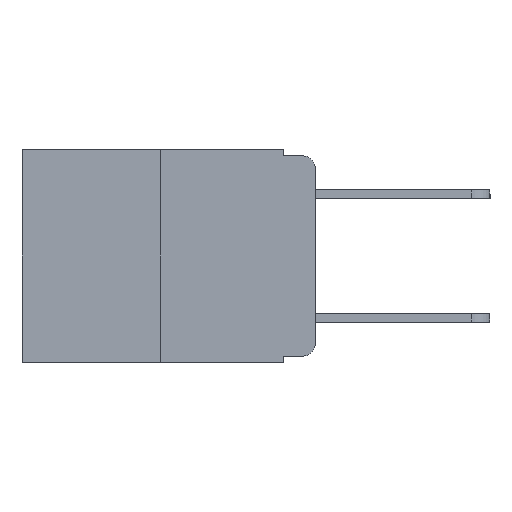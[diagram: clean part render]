
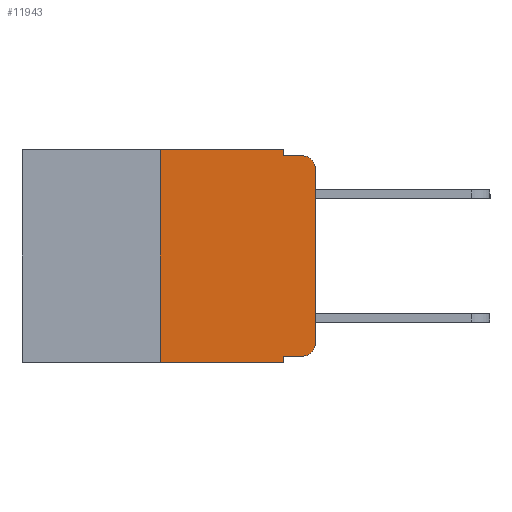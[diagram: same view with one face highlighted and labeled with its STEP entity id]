
A CAD part, left-side view. The second image highlights one B-rep face of the part: STEP entity #11943.
In plain terms, the highlighted planar face has unit normal (-1, 0, 0).
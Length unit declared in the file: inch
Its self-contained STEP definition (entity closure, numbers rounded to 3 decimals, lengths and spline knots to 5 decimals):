
#46 = ORIENTED_EDGE ( 'NONE', *, *, #11764, .F. ) ;
#223 = CARTESIAN_POINT ( 'NONE',  ( 0., 0.02, -0.313 ) ) ;
#431 = CARTESIAN_POINT ( 'NONE',  ( 0., 0.25, 0. ) ) ;
#794 = DIRECTION ( 'NONE',  ( -1., 0., 0. ) ) ;
#873 = ORIENTED_EDGE ( 'NONE', *, *, #11497, .T. ) ;
#1015 = CARTESIAN_POINT ( 'NONE',  ( 0., 0.051, -0.333 ) ) ;
#1298 = DIRECTION ( 'NONE',  ( 0., 0., -1. ) ) ;
#1335 = DIRECTION ( 'NONE',  ( 1., 0., 0. ) ) ;
#1840 = CARTESIAN_POINT ( 'NONE',  ( 0., 0.051, -0.01 ) ) ;
#1846 = ORIENTED_EDGE ( 'NONE', *, *, #12271, .F. ) ;
#1967 = VERTEX_POINT ( 'NONE', #11805 ) ;
#2085 = VERTEX_POINT ( 'NONE', #2426 ) ;
#2142 = VECTOR ( 'NONE', #12217, 39.37008 ) ;
#2426 = CARTESIAN_POINT ( 'NONE',  ( 0., 0.02, -0.333 ) ) ;
#2432 = VERTEX_POINT ( 'NONE', #2694 ) ;
#2457 = CARTESIAN_POINT ( 'NONE',  ( 0., 0.051, -0.333 ) ) ;
#2475 = LINE ( 'NONE', #9108, #10427 ) ;
#2492 = CARTESIAN_POINT ( 'NONE',  ( 0., 0.25, -0.343 ) ) ;
#2615 = EDGE_CURVE ( 'NONE', #10436, #3575, #9193, .T. ) ;
#2694 = CARTESIAN_POINT ( 'NONE',  ( 0., 0.02, -0.01 ) ) ;
#2978 = LINE ( 'NONE', #10700, #7921 ) ;
#3047 = VECTOR ( 'NONE', #7448, 39.37008 ) ;
#3259 = EDGE_CURVE ( 'NONE', #6169, #12086, #2475, .T. ) ;
#3275 = EDGE_CURVE ( 'NONE', #6140, #1967, #9878, .T. ) ;
#3575 = VERTEX_POINT ( 'NONE', #10902 ) ;
#3924 = EDGE_LOOP ( 'NONE', ( #873, #11348, #1846, #7428, #46, #10440, #8321, #6031, #8918, #6675 ) ) ;
#4031 = DIRECTION ( 'NONE',  ( 0., -1., 0. ) ) ;
#4522 = DIRECTION ( 'NONE',  ( 0., 0., -1. ) ) ;
#4551 = EDGE_CURVE ( 'NONE', #6140, #2085, #8284, .T. ) ;
#4574 = CARTESIAN_POINT ( 'NONE',  ( 0., 0.473, -0.343 ) ) ;
#4646 = CIRCLE ( 'NONE', #7468, 0.02 ) ;
#4783 = DIRECTION ( 'NONE',  ( 0., -1., 0. ) ) ;
#4808 = EDGE_CURVE ( 'NONE', #2085, #6910, #11317, .T. ) ;
#5000 = AXIS2_PLACEMENT_3D ( 'NONE', #223, #7238, #1298 ) ;
#5977 = DIRECTION ( 'NONE',  ( 0., -1., 0. ) ) ;
#5992 = VECTOR ( 'NONE', #5977, 39.37008 ) ;
#6031 = ORIENTED_EDGE ( 'NONE', *, *, #3275, .F. ) ;
#6140 = VERTEX_POINT ( 'NONE', #2457 ) ;
#6169 = VERTEX_POINT ( 'NONE', #2492 ) ;
#6469 = CARTESIAN_POINT ( 'NONE',  ( 0., 0., 0. ) ) ;
#6496 = CARTESIAN_POINT ( 'NONE',  ( 0., 0., -0.313 ) ) ;
#6675 = ORIENTED_EDGE ( 'NONE', *, *, #4808, .T. ) ;
#6736 = FACE_OUTER_BOUND ( 'NONE', #3924, .T. ) ;
#6776 = CARTESIAN_POINT ( 'NONE',  ( 0., 0.051, 0. ) ) ;
#6801 = CARTESIAN_POINT ( 'NONE',  ( 0., 0.02, -0.03 ) ) ;
#6910 = VERTEX_POINT ( 'NONE', #6496 ) ;
#6925 = CARTESIAN_POINT ( 'NONE',  ( 0., 0., -0.03 ) ) ;
#7024 = VECTOR ( 'NONE', #4783, 39.37008 ) ;
#7238 = DIRECTION ( 'NONE',  ( -1., 0., 0. ) ) ;
#7245 = VERTEX_POINT ( 'NONE', #6925 ) ;
#7428 = ORIENTED_EDGE ( 'NONE', *, *, #2615, .F. ) ;
#7448 = DIRECTION ( 'NONE',  ( 0., 0., 1. ) ) ;
#7468 = AXIS2_PLACEMENT_3D ( 'NONE', #6801, #794, #7768 ) ;
#7676 = CARTESIAN_POINT ( 'NONE',  ( 0., 0.051, 0. ) ) ;
#7768 = DIRECTION ( 'NONE',  ( 0., 0., -1. ) ) ;
#7921 = VECTOR ( 'NONE', #4031, 39.37008 ) ;
#8131 = CARTESIAN_POINT ( 'NONE',  ( 0., 0.051, 0. ) ) ;
#8234 = DIRECTION ( 'NONE',  ( 0., 0., -1. ) ) ;
#8284 = LINE ( 'NONE', #1015, #5992 ) ;
#8321 = ORIENTED_EDGE ( 'NONE', *, *, #10077, .T. ) ;
#8918 = ORIENTED_EDGE ( 'NONE', *, *, #4551, .T. ) ;
#8977 = AXIS2_PLACEMENT_3D ( 'NONE', #9142, #1335, #8234 ) ;
#9108 = CARTESIAN_POINT ( 'NONE',  ( 0., 0.25, 0. ) ) ;
#9142 = CARTESIAN_POINT ( 'NONE',  ( 0., 0.473, 0. ) ) ;
#9193 = LINE ( 'NONE', #7676, #11198 ) ;
#9541 = LINE ( 'NONE', #1840, #7024 ) ;
#9636 = VECTOR ( 'NONE', #11160, 39.37008 ) ;
#9878 = LINE ( 'NONE', #6776, #2142 ) ;
#10077 = EDGE_CURVE ( 'NONE', #6169, #1967, #12121, .T. ) ;
#10427 = VECTOR ( 'NONE', #11551, 39.37008 ) ;
#10436 = VERTEX_POINT ( 'NONE', #8131 ) ;
#10440 = ORIENTED_EDGE ( 'NONE', *, *, #3259, .F. ) ;
#10678 = LINE ( 'NONE', #6469, #3047 ) ;
#10700 = CARTESIAN_POINT ( 'NONE',  ( 0., 0.473, 0. ) ) ;
#10869 = PLANE ( 'NONE',  #8977 ) ;
#10902 = CARTESIAN_POINT ( 'NONE',  ( 0., 0.051, -0.01 ) ) ;
#11160 = DIRECTION ( 'NONE',  ( 0., -1., 0. ) ) ;
#11198 = VECTOR ( 'NONE', #4522, 39.37008 ) ;
#11317 = CIRCLE ( 'NONE', #5000, 0.02 ) ;
#11348 = ORIENTED_EDGE ( 'NONE', *, *, #12253, .T. ) ;
#11497 = EDGE_CURVE ( 'NONE', #6910, #7245, #10678, .T. ) ;
#11551 = DIRECTION ( 'NONE',  ( 0., 0., 1. ) ) ;
#11764 = EDGE_CURVE ( 'NONE', #12086, #10436, #2978, .T. ) ;
#11805 = CARTESIAN_POINT ( 'NONE',  ( 0., 0.051, -0.343 ) ) ;
#11943 = ADVANCED_FACE ( 'NONE', ( #6736 ), #10869, .F. ) ;
#12086 = VERTEX_POINT ( 'NONE', #431 ) ;
#12121 = LINE ( 'NONE', #4574, #9636 ) ;
#12217 = DIRECTION ( 'NONE',  ( 0., 0., -1. ) ) ;
#12253 = EDGE_CURVE ( 'NONE', #7245, #2432, #4646, .T. ) ;
#12271 = EDGE_CURVE ( 'NONE', #3575, #2432, #9541, .T. ) ;
